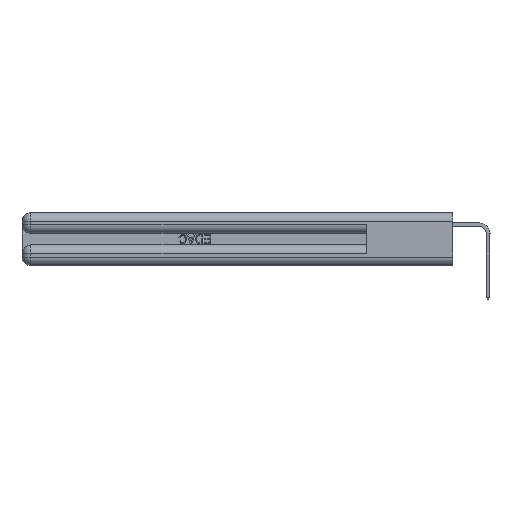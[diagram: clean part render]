
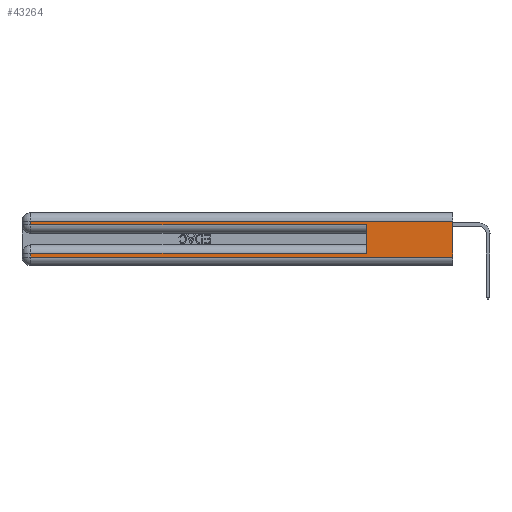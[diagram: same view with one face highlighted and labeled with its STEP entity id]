
A CAD part, left-side view. The second image highlights one B-rep face of the part: STEP entity #43264.
In plain terms, the highlighted planar face has unit normal (-1, 0, 0).
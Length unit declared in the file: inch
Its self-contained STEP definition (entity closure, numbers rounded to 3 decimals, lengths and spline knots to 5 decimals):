
#1 = ORIENTED_EDGE ( 'NONE', *, *, #47027, .F. ) ;
#4618 = DIRECTION ( 'NONE',  ( 0., 0., -1. ) ) ;
#4964 = VECTOR ( 'NONE', #16507, 39.37008 ) ;
#5116 = LINE ( 'NONE', #20705, #37523 ) ;
#6105 = CARTESIAN_POINT ( 'NONE',  ( 0., 0., 0.06 ) ) ;
#6673 = VECTOR ( 'NONE', #37278, 39.37008 ) ;
#7237 = CARTESIAN_POINT ( 'NONE',  ( 0., 0., 0.31 ) ) ;
#7903 = EDGE_CURVE ( 'NONE', #36950, #11078, #41174, .T. ) ;
#8104 = VERTEX_POINT ( 'NONE', #44896 ) ;
#9233 = DIRECTION ( 'NONE',  ( 1., 0., 0. ) ) ;
#11078 = VERTEX_POINT ( 'NONE', #13660 ) ;
#12009 = CARTESIAN_POINT ( 'NONE',  ( 0., 0., 0.285 ) ) ;
#12263 = CARTESIAN_POINT ( 'NONE',  ( 0., 0., 0.06 ) ) ;
#13272 = CARTESIAN_POINT ( 'NONE',  ( 0., 2.94, 0.06 ) ) ;
#13660 = CARTESIAN_POINT ( 'NONE',  ( 0., 2.94, 0.085 ) ) ;
#14621 = DIRECTION ( 'NONE',  ( 0., 0., 1. ) ) ;
#15572 = ORIENTED_EDGE ( 'NONE', *, *, #34210, .T. ) ;
#16507 = DIRECTION ( 'NONE',  ( 0., -1., 0. ) ) ;
#17071 = CARTESIAN_POINT ( 'NONE',  ( 0., 0., 0.31 ) ) ;
#17097 = LINE ( 'NONE', #7237, #26955 ) ;
#19036 = EDGE_CURVE ( 'NONE', #28924, #19586, #17097, .T. ) ;
#19586 = VERTEX_POINT ( 'NONE', #36163 ) ;
#20705 = CARTESIAN_POINT ( 'NONE',  ( 0., 2.94, 0.37 ) ) ;
#20744 = EDGE_CURVE ( 'NONE', #11078, #38001, #30737, .T. ) ;
#20945 = FACE_OUTER_BOUND ( 'NONE', #46945, .T. ) ;
#21126 = ORIENTED_EDGE ( 'NONE', *, *, #26214, .T. ) ;
#21665 = ORIENTED_EDGE ( 'NONE', *, *, #20744, .T. ) ;
#22369 = CARTESIAN_POINT ( 'NONE',  ( 0., 0., 0.085 ) ) ;
#23496 = CARTESIAN_POINT ( 'NONE',  ( 0., 0.6, 0.085 ) ) ;
#24194 = DIRECTION ( 'NONE',  ( 0., 1., 0. ) ) ;
#24930 = DIRECTION ( 'NONE',  ( 0., 0., -1. ) ) ;
#25944 = VERTEX_POINT ( 'NONE', #6105 ) ;
#26214 = EDGE_CURVE ( 'NONE', #19586, #43778, #5116, .T. ) ;
#26618 = DIRECTION ( 'NONE',  ( 0., 1., 0. ) ) ;
#26955 = VECTOR ( 'NONE', #24194, 39.37008 ) ;
#28642 = VECTOR ( 'NONE', #26618, 39.37008 ) ;
#28924 = VERTEX_POINT ( 'NONE', #17071 ) ;
#30737 = LINE ( 'NONE', #40301, #40640 ) ;
#31218 = ORIENTED_EDGE ( 'NONE', *, *, #37170, .T. ) ;
#31399 = CARTESIAN_POINT ( 'NONE',  ( 0., 0.6, 0.145 ) ) ;
#32380 = CARTESIAN_POINT ( 'NONE',  ( 0., 2.94, 0.285 ) ) ;
#34210 = EDGE_CURVE ( 'NONE', #43778, #8104, #40380, .T. ) ;
#34231 = CARTESIAN_POINT ( 'NONE',  ( 0., 0., 0.37 ) ) ;
#34356 = LINE ( 'NONE', #31399, #54165 ) ;
#34371 = PLANE ( 'NONE',  #54685 ) ;
#34554 = CARTESIAN_POINT ( 'NONE',  ( 0., 0., 0.37 ) ) ;
#36163 = CARTESIAN_POINT ( 'NONE',  ( 0., 2.94, 0.31 ) ) ;
#36950 = VERTEX_POINT ( 'NONE', #23496 ) ;
#37170 = EDGE_CURVE ( 'NONE', #38001, #25944, #38671, .T. ) ;
#37278 = DIRECTION ( 'NONE',  ( 0., -1., 0. ) ) ;
#37350 = VECTOR ( 'NONE', #4618, 39.37008 ) ;
#37523 = VECTOR ( 'NONE', #24930, 39.37008 ) ;
#38001 = VERTEX_POINT ( 'NONE', #13272 ) ;
#38671 = LINE ( 'NONE', #12263, #4964 ) ;
#38752 = DIRECTION ( 'NONE',  ( 0., 0., -1. ) ) ;
#40301 = CARTESIAN_POINT ( 'NONE',  ( 0., 2.94, 0.37 ) ) ;
#40380 = LINE ( 'NONE', #12009, #6673 ) ;
#40640 = VECTOR ( 'NONE', #44550, 39.37008 ) ;
#41174 = LINE ( 'NONE', #22369, #28642 ) ;
#43264 = ADVANCED_FACE ( 'NONE', ( #20945 ), #34371, .F. ) ;
#43778 = VERTEX_POINT ( 'NONE', #32380 ) ;
#44032 = EDGE_CURVE ( 'NONE', #28924, #25944, #49937, .T. ) ;
#44134 = ORIENTED_EDGE ( 'NONE', *, *, #44032, .F. ) ;
#44550 = DIRECTION ( 'NONE',  ( 0., 0., -1. ) ) ;
#44831 = ORIENTED_EDGE ( 'NONE', *, *, #7903, .T. ) ;
#44896 = CARTESIAN_POINT ( 'NONE',  ( 0., 0.6, 0.285 ) ) ;
#46945 = EDGE_LOOP ( 'NONE', ( #44134, #52143, #21126, #15572, #1, #44831, #21665, #31218 ) ) ;
#47027 = EDGE_CURVE ( 'NONE', #36950, #8104, #34356, .T. ) ;
#49937 = LINE ( 'NONE', #34231, #37350 ) ;
#52143 = ORIENTED_EDGE ( 'NONE', *, *, #19036, .T. ) ;
#54165 = VECTOR ( 'NONE', #14621, 39.37008 ) ;
#54685 = AXIS2_PLACEMENT_3D ( 'NONE', #34554, #9233, #38752 ) ;
